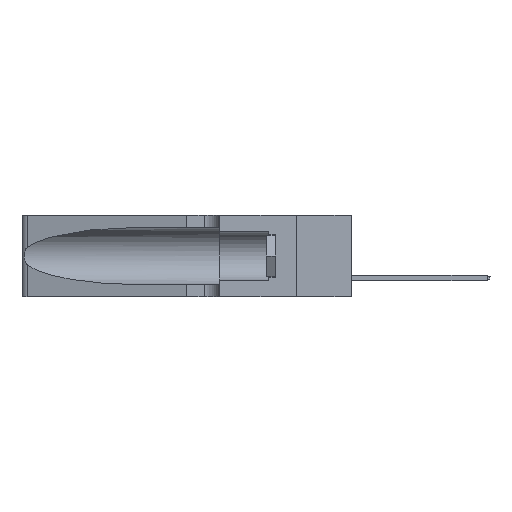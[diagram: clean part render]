
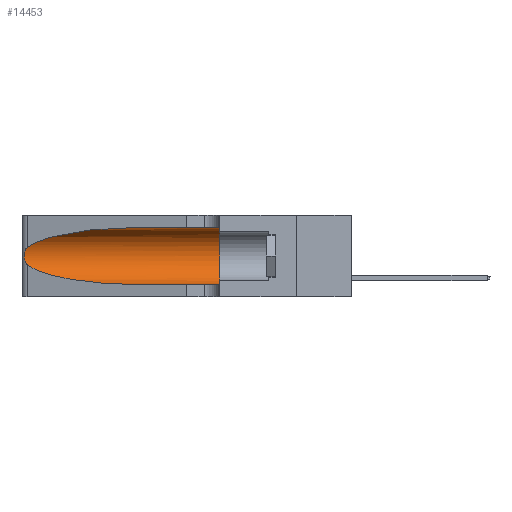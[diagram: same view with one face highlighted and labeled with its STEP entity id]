
A CAD part, left-side view. The second image highlights one B-rep face of the part: STEP entity #14453.
In plain terms, the highlighted cylindrical face has radius 3.308 mm (diameter 6.617 mm), a partial arc.
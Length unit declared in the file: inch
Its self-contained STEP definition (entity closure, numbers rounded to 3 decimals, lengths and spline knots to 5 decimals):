
#204 = EDGE_CURVE ( 'NONE', #18060, #26037, #24219, .T. ) ;
#889 = CARTESIAN_POINT ( 'NONE',  ( 0.1305, 0.72297, 0.31525 ) ) ;
#4110 = CARTESIAN_POINT ( 'NONE',  ( 0.2373, 1.15595, 0.08982 ) ) ;
#4164 = CARTESIAN_POINT ( 'NONE',  ( 0.25787, 1.23484, 0.2124 ) ) ;
#4501 = FACE_OUTER_BOUND ( 'NONE', #13703, .T. ) ;
#4526 = CARTESIAN_POINT ( 'NONE',  ( 0.25789, 1.23486, 0.15765 ) ) ;
#4652 = B_SPLINE_CURVE_WITH_KNOTS ( 'NONE', 3,
 ( #8527, #19465, #13076, #4164, #26266, #21661, #25880, #10791, #17194, #24039, #4526, #19567, #21756, #26074 ),
 .UNSPECIFIED., .F., .F.,
 ( 4, 2, 2, 2, 2, 2, 4 ),
 ( 0., 0.00027, 0.00053, 0.00107, 0.0016, 0.00187, 0.00214 ),
 .UNSPECIFIED. ) ;
#6259 = ORIENTED_EDGE ( 'NONE', *, *, #22998, .T. ) ;
#6362 = ORIENTED_EDGE ( 'NONE', *, *, #8762, .T. ) ;
#7052 = ORIENTED_EDGE ( 'NONE', *, *, #204, .T. ) ;
#7539 = DIRECTION ( 'NONE',  ( 0., 0., -1. ) ) ;
#7821 = CARTESIAN_POINT ( 'NONE',  ( 0.1305, 0.72297, 0.05475 ) ) ;
#8527 = CARTESIAN_POINT ( 'NONE',  ( 0.25487, 1.22718, 0.22369 ) ) ;
#8762 = EDGE_CURVE ( 'NONE', #11869, #14879, #9039, .T. ) ;
#8900 = DIRECTION ( 'NONE',  ( 0., -1., 0. ) ) ;
#8971 = CARTESIAN_POINT ( 'NONE',  ( 0.25487, 1.22718, 0.14631 ) ) ;
#9039 =( BOUNDED_CURVE ( )  B_SPLINE_CURVE ( 3, ( #889, #25462, #21034, #12093 ),
 .UNSPECIFIED., .F., .F. ) 
 B_SPLINE_CURVE_WITH_KNOTS ( ( 4, 4 ),
 ( 1.5708, 2.84003 ),
 .UNSPECIFIED. ) 
 CURVE ( )  GEOMETRIC_REPRESENTATION_ITEM ( )  RATIONAL_B_SPLINE_CURVE ( ( 1., 0.87, 0.87, 1. ) ) 
 REPRESENTATION_ITEM ( '' )  );
#9335 = CARTESIAN_POINT ( 'NONE',  ( 0.1305, 0.35, 0.05475 ) ) ;
#9404 = ORIENTED_EDGE ( 'NONE', *, *, #25732, .F. ) ;
#9546 = CARTESIAN_POINT ( 'NONE',  ( 0.1305, 1.61858, 0.185 ) ) ;
#9911 = EDGE_CURVE ( 'NONE', #21637, #14204, #11573, .T. ) ;
#10408 = ORIENTED_EDGE ( 'NONE', *, *, #9911, .F. ) ;
#10739 = VECTOR ( 'NONE', #26545, 39.37008 ) ;
#10791 = CARTESIAN_POINT ( 'NONE',  ( 0.26075, 1.23896, 0.178 ) ) ;
#11142 = CARTESIAN_POINT ( 'NONE',  ( 0.1305, 0.35, 0.31525 ) ) ;
#11573 = CIRCLE ( 'NONE', #18766, 0.13025 ) ;
#11869 = VERTEX_POINT ( 'NONE', #20393 ) ;
#12093 = CARTESIAN_POINT ( 'NONE',  ( 0.25487, 1.22718, 0.22369 ) ) ;
#13076 = CARTESIAN_POINT ( 'NONE',  ( 0.25639, 1.23184, 0.21858 ) ) ;
#13112 = CARTESIAN_POINT ( 'NONE',  ( 0.18966, 0.96281, 0.05475 ) ) ;
#13703 = EDGE_LOOP ( 'NONE', ( #6362, #25178, #7052, #6259, #10408, #9404 ) ) ;
#14204 = VERTEX_POINT ( 'NONE', #9335 ) ;
#14453 = ADVANCED_FACE ( 'NONE', ( #4501 ), #19147, .F. ) ;
#14879 = VERTEX_POINT ( 'NONE', #24379 ) ;
#17194 = CARTESIAN_POINT ( 'NONE',  ( 0.26017, 1.23833, 0.17102 ) ) ;
#18060 = VERTEX_POINT ( 'NONE', #8971 ) ;
#18766 = AXIS2_PLACEMENT_3D ( 'NONE', #24044, #21859, #20044 ) ;
#19147 = CYLINDRICAL_SURFACE ( 'NONE', #26336, 0.13025 ) ;
#19321 = CARTESIAN_POINT ( 'NONE',  ( 0.25487, 1.22718, 0.14631 ) ) ;
#19416 = CARTESIAN_POINT ( 'NONE',  ( 0.1305, 0.72297, 0.05475 ) ) ;
#19465 = CARTESIAN_POINT ( 'NONE',  ( 0.25555, 1.22994, 0.2215 ) ) ;
#19567 = CARTESIAN_POINT ( 'NONE',  ( 0.25639, 1.23186, 0.15144 ) ) ;
#19836 = LINE ( 'NONE', #24132, #28050 ) ;
#20044 = DIRECTION ( 'NONE',  ( 0., 0., 1. ) ) ;
#20393 = CARTESIAN_POINT ( 'NONE',  ( 0.1305, 0.72297, 0.31525 ) ) ;
#20634 = LINE ( 'NONE', #25480, #10739 ) ;
#21034 = CARTESIAN_POINT ( 'NONE',  ( 0.2373, 1.15595, 0.28018 ) ) ;
#21637 = VERTEX_POINT ( 'NONE', #11142 ) ;
#21661 = CARTESIAN_POINT ( 'NONE',  ( 0.26018, 1.23835, 0.19895 ) ) ;
#21756 = CARTESIAN_POINT ( 'NONE',  ( 0.25555, 1.22993, 0.14849 ) ) ;
#21859 = DIRECTION ( 'NONE',  ( 0., 1., 0. ) ) ;
#22998 = EDGE_CURVE ( 'NONE', #26037, #14204, #20634, .T. ) ;
#24039 = CARTESIAN_POINT ( 'NONE',  ( 0.25856, 1.23593, 0.16098 ) ) ;
#24044 = CARTESIAN_POINT ( 'NONE',  ( 0.1305, 0.35, 0.185 ) ) ;
#24132 = CARTESIAN_POINT ( 'NONE',  ( 0.1305, 1.61858, 0.31525 ) ) ;
#24219 =( BOUNDED_CURVE ( )  B_SPLINE_CURVE ( 3, ( #19321, #4110, #13112, #19416 ),
 .UNSPECIFIED., .F., .T. ) 
 B_SPLINE_CURVE_WITH_KNOTS ( ( 4, 4 ),
 ( 3.44316, 4.71239 ),
 .UNSPECIFIED. ) 
 CURVE ( )  GEOMETRIC_REPRESENTATION_ITEM ( )  RATIONAL_B_SPLINE_CURVE ( ( 1., 0.87, 0.87, 1. ) ) 
 REPRESENTATION_ITEM ( '' )  );
#24379 = CARTESIAN_POINT ( 'NONE',  ( 0.25487, 1.22718, 0.22369 ) ) ;
#24718 = EDGE_CURVE ( 'NONE', #14879, #18060, #4652, .T. ) ;
#25178 = ORIENTED_EDGE ( 'NONE', *, *, #24718, .T. ) ;
#25462 = CARTESIAN_POINT ( 'NONE',  ( 0.18966, 0.96281, 0.31525 ) ) ;
#25480 = CARTESIAN_POINT ( 'NONE',  ( 0.1305, 1.61858, 0.05475 ) ) ;
#25732 = EDGE_CURVE ( 'NONE', #11869, #21637, #19836, .T. ) ;
#25880 = CARTESIAN_POINT ( 'NONE',  ( 0.26075, 1.23896, 0.19203 ) ) ;
#26037 = VERTEX_POINT ( 'NONE', #7821 ) ;
#26074 = CARTESIAN_POINT ( 'NONE',  ( 0.25487, 1.22718, 0.14631 ) ) ;
#26266 = CARTESIAN_POINT ( 'NONE',  ( 0.25854, 1.2359, 0.20912 ) ) ;
#26336 = AXIS2_PLACEMENT_3D ( 'NONE', #9546, #27119, #7539 ) ;
#26545 = DIRECTION ( 'NONE',  ( 0., -1., 0. ) ) ;
#27119 = DIRECTION ( 'NONE',  ( 0., -1., 0. ) ) ;
#28050 = VECTOR ( 'NONE', #8900, 39.37008 ) ;
